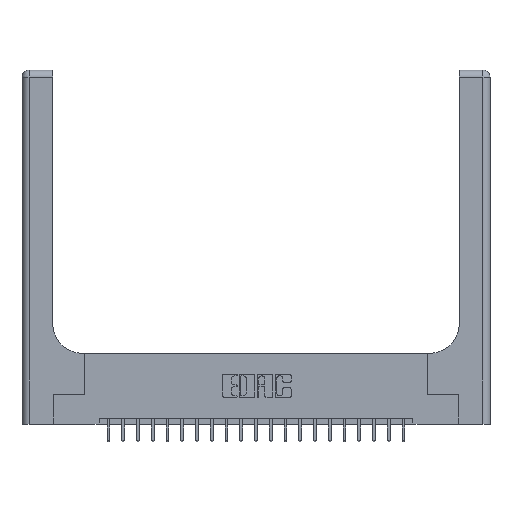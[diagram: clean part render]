
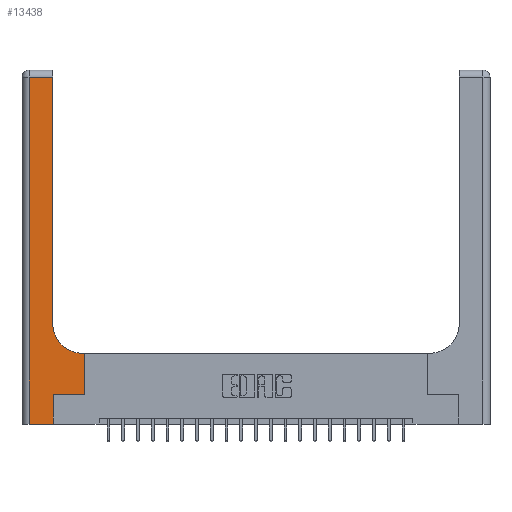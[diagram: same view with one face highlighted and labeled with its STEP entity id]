
A CAD part, top view. The second image highlights one B-rep face of the part: STEP entity #13438.
In plain terms, the highlighted planar face has unit normal (0, 0, 1).
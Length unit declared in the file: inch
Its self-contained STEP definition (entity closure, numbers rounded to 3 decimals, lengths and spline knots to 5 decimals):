
#212 = DIRECTION ( 'NONE',  ( 1., 0., 0. ) ) ;
#1122 = CARTESIAN_POINT ( 'NONE',  ( 0., 2.94, 0.37 ) ) ;
#1390 = CARTESIAN_POINT ( 'NONE',  ( 0.265, 0., 0.37 ) ) ;
#2122 = DIRECTION ( 'NONE',  ( 1., 0., 0. ) ) ;
#2590 = VECTOR ( 'NONE', #2716, 39.37008 ) ;
#2716 = DIRECTION ( 'NONE',  ( 0., 1., 0. ) ) ;
#3466 = VECTOR ( 'NONE', #15808, 39.37008 ) ;
#4091 = VERTEX_POINT ( 'NONE', #16925 ) ;
#4225 = ORIENTED_EDGE ( 'NONE', *, *, #16753, .T. ) ;
#4356 = CARTESIAN_POINT ( 'NONE',  ( 0.265, 0.25, 0.37 ) ) ;
#4489 = VERTEX_POINT ( 'NONE', #9631 ) ;
#4686 = DIRECTION ( 'NONE',  ( 0., 1., 0. ) ) ;
#4715 = ORIENTED_EDGE ( 'NONE', *, *, #17512, .T. ) ;
#4833 = CARTESIAN_POINT ( 'NONE',  ( 0.265, 0., 0.37 ) ) ;
#4866 = CARTESIAN_POINT ( 'NONE',  ( 0., 0., 0.37 ) ) ;
#5695 = CARTESIAN_POINT ( 'NONE',  ( 0.06, 0., 0.37 ) ) ;
#6055 = VERTEX_POINT ( 'NONE', #5695 ) ;
#6274 = LINE ( 'NONE', #17132, #13571 ) ;
#6329 = CARTESIAN_POINT ( 'NONE',  ( 0.528, 0.6, 0.37 ) ) ;
#6352 = CARTESIAN_POINT ( 'NONE',  ( 0., 3., 0.37 ) ) ;
#6904 = VECTOR ( 'NONE', #13688, 39.37008 ) ;
#6955 = DIRECTION ( 'NONE',  ( 0., 1., 0. ) ) ;
#7238 = LINE ( 'NONE', #4866, #8283 ) ;
#7590 = LINE ( 'NONE', #19462, #2590 ) ;
#7707 = CARTESIAN_POINT ( 'NONE',  ( 0.06, 2.94, 0.37 ) ) ;
#7888 = VERTEX_POINT ( 'NONE', #4356 ) ;
#8283 = VECTOR ( 'NONE', #212, 39.37008 ) ;
#8591 = VERTEX_POINT ( 'NONE', #1390 ) ;
#9513 = CARTESIAN_POINT ( 'NONE',  ( 0.26, 0.6, 0.37 ) ) ;
#9515 = ORIENTED_EDGE ( 'NONE', *, *, #10628, .T. ) ;
#9607 = CIRCLE ( 'NONE', #10997, 0.25 ) ;
#9631 = CARTESIAN_POINT ( 'NONE',  ( 0.26, 0.85, 0.37 ) ) ;
#9929 = DIRECTION ( 'NONE',  ( -1., 0., 0. ) ) ;
#10101 = VERTEX_POINT ( 'NONE', #7707 ) ;
#10505 = VERTEX_POINT ( 'NONE', #6329 ) ;
#10618 = CARTESIAN_POINT ( 'NONE',  ( 0.528, 0.25, 0.37 ) ) ;
#10628 = EDGE_CURVE ( 'NONE', #10505, #11200, #12331, .T. ) ;
#10997 = AXIS2_PLACEMENT_3D ( 'NONE', #20631, #13770, #2122 ) ;
#11146 = EDGE_CURVE ( 'NONE', #4489, #4091, #7590, .T. ) ;
#11200 = VERTEX_POINT ( 'NONE', #19688 ) ;
#11504 = EDGE_CURVE ( 'NONE', #11754, #10505, #6274, .T. ) ;
#11728 = VECTOR ( 'NONE', #14500, 39.37008 ) ;
#11754 = VERTEX_POINT ( 'NONE', #10618 ) ;
#11993 = CARTESIAN_POINT ( 'NONE',  ( 0.265, 0.25, 0.37 ) ) ;
#12331 = LINE ( 'NONE', #9513, #13622 ) ;
#12885 = EDGE_CURVE ( 'NONE', #4091, #10101, #19101, .T. ) ;
#13138 = DIRECTION ( 'NONE',  ( 0., 0., -1. ) ) ;
#13438 = ADVANCED_FACE ( 'NONE', ( #21220 ), #19851, .F. ) ;
#13571 = VECTOR ( 'NONE', #6955, 39.37008 ) ;
#13622 = VECTOR ( 'NONE', #17926, 39.37008 ) ;
#13688 = DIRECTION ( 'NONE',  ( 1., 0., 0. ) ) ;
#13770 = DIRECTION ( 'NONE',  ( 0., 0., -1. ) ) ;
#14004 = ORIENTED_EDGE ( 'NONE', *, *, #12885, .T. ) ;
#14264 = LINE ( 'NONE', #4833, #17698 ) ;
#14275 = EDGE_LOOP ( 'NONE', ( #18980, #14004, #4715, #18121, #17353, #4225, #16458, #9515, #17869 ) ) ;
#14415 = EDGE_CURVE ( 'NONE', #11200, #4489, #9607, .T. ) ;
#14426 = EDGE_CURVE ( 'NONE', #6055, #8591, #7238, .T. ) ;
#14500 = DIRECTION ( 'NONE',  ( -1., 0., 0. ) ) ;
#15292 = EDGE_CURVE ( 'NONE', #8591, #7888, #14264, .T. ) ;
#15808 = DIRECTION ( 'NONE',  ( 0., -1., 0. ) ) ;
#16458 = ORIENTED_EDGE ( 'NONE', *, *, #11504, .T. ) ;
#16687 = AXIS2_PLACEMENT_3D ( 'NONE', #6352, #13138, #9929 ) ;
#16753 = EDGE_CURVE ( 'NONE', #7888, #11754, #20303, .T. ) ;
#16808 = LINE ( 'NONE', #20839, #3466 ) ;
#16925 = CARTESIAN_POINT ( 'NONE',  ( 0.26, 2.94, 0.37 ) ) ;
#17132 = CARTESIAN_POINT ( 'NONE',  ( 0.528, 0.25, 0.37 ) ) ;
#17353 = ORIENTED_EDGE ( 'NONE', *, *, #15292, .T. ) ;
#17512 = EDGE_CURVE ( 'NONE', #10101, #6055, #16808, .T. ) ;
#17698 = VECTOR ( 'NONE', #4686, 39.37008 ) ;
#17869 = ORIENTED_EDGE ( 'NONE', *, *, #14415, .T. ) ;
#17926 = DIRECTION ( 'NONE',  ( -1., 0., 0. ) ) ;
#18121 = ORIENTED_EDGE ( 'NONE', *, *, #14426, .T. ) ;
#18980 = ORIENTED_EDGE ( 'NONE', *, *, #11146, .T. ) ;
#19101 = LINE ( 'NONE', #1122, #11728 ) ;
#19462 = CARTESIAN_POINT ( 'NONE',  ( 0.26, 3., 0.37 ) ) ;
#19688 = CARTESIAN_POINT ( 'NONE',  ( 0.51, 0.6, 0.37 ) ) ;
#19851 = PLANE ( 'NONE',  #16687 ) ;
#20303 = LINE ( 'NONE', #11993, #6904 ) ;
#20631 = CARTESIAN_POINT ( 'NONE',  ( 0.51, 0.85, 0.37 ) ) ;
#20839 = CARTESIAN_POINT ( 'NONE',  ( 0.06, 3., 0.37 ) ) ;
#21220 = FACE_OUTER_BOUND ( 'NONE', #14275, .T. ) ;
